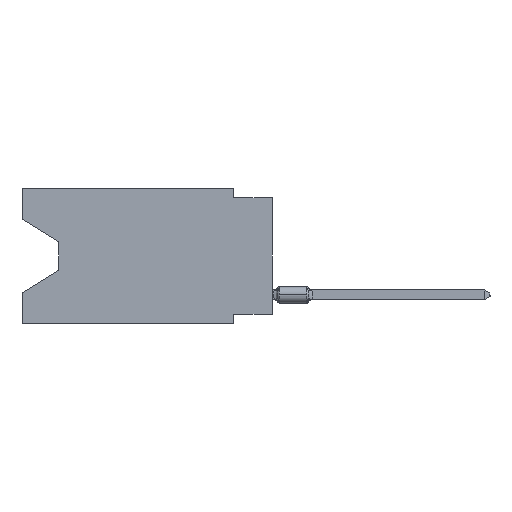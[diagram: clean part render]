
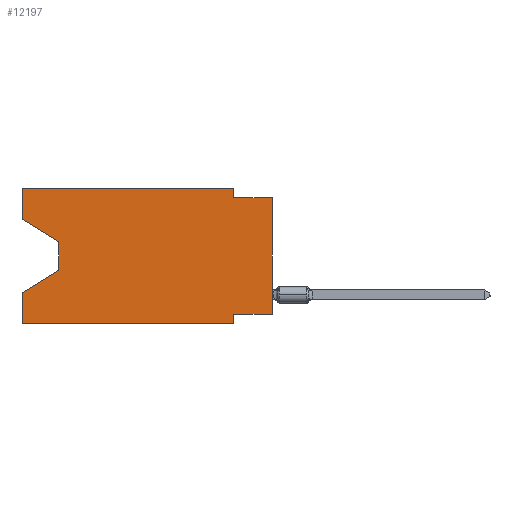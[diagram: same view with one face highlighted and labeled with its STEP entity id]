
A CAD part, left-side view. The second image highlights one B-rep face of the part: STEP entity #12197.
In plain terms, the highlighted planar face has unit normal (-1, 0, 0).
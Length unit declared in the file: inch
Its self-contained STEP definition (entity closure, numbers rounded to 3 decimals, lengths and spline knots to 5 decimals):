
#120 = CARTESIAN_POINT ( 'NONE',  ( 0., 0.645, 0. ) ) ;
#239 = VERTEX_POINT ( 'NONE', #30306 ) ;
#517 = FACE_OUTER_BOUND ( 'NONE', #9209, .T. ) ;
#869 = ORIENTED_EDGE ( 'NONE', *, *, #15282, .T. ) ;
#912 = DIRECTION ( 'NONE',  ( 0., 1., 0. ) ) ;
#1677 = DIRECTION ( 'NONE',  ( 0., 0., -1. ) ) ;
#1765 = VECTOR ( 'NONE', #13354, 39.37008 ) ;
#1964 = CARTESIAN_POINT ( 'NONE',  ( 0., 0.645, -0.08025 ) ) ;
#2589 = ORIENTED_EDGE ( 'NONE', *, *, #3923, .F. ) ;
#2932 = DIRECTION ( 'NONE',  ( 0., 0., 1. ) ) ;
#3113 = DIRECTION ( 'NONE',  ( 1., 0., 0. ) ) ;
#3173 = ORIENTED_EDGE ( 'NONE', *, *, #23445, .T. ) ;
#3202 = CARTESIAN_POINT ( 'NONE',  ( 0., 0.645, 0. ) ) ;
#3367 = LINE ( 'NONE', #14789, #26291 ) ;
#3440 = EDGE_CURVE ( 'NONE', #21007, #14443, #19970, .T. ) ;
#3761 = VECTOR ( 'NONE', #20895, 39.37008 ) ;
#3923 = EDGE_CURVE ( 'NONE', #27472, #8868, #16144, .T. ) ;
#5024 = ORIENTED_EDGE ( 'NONE', *, *, #17953, .T. ) ;
#5385 = CARTESIAN_POINT ( 'NONE',  ( 0., 0.1, -0.35 ) ) ;
#6150 = LINE ( 'NONE', #11535, #6259 ) ;
#6226 = CARTESIAN_POINT ( 'NONE',  ( 0., 0.55, -0.212 ) ) ;
#6236 = VECTOR ( 'NONE', #27005, 39.37008 ) ;
#6259 = VECTOR ( 'NONE', #1677, 39.37008 ) ;
#6413 = DIRECTION ( 'NONE',  ( 0., -1., 0. ) ) ;
#7606 = LINE ( 'NONE', #14845, #24814 ) ;
#8752 = VERTEX_POINT ( 'NONE', #9544 ) ;
#8868 = VERTEX_POINT ( 'NONE', #14634 ) ;
#9046 = DIRECTION ( 'NONE',  ( 0., -0.855, -0.519 ) ) ;
#9209 = EDGE_LOOP ( 'NONE', ( #3173, #12405, #17826, #14183, #869, #27420, #13983, #5024, #28191, #11538, #2589, #18697 ) ) ;
#9544 = CARTESIAN_POINT ( 'NONE',  ( 0., 0.1, -0.325 ) ) ;
#9711 = EDGE_CURVE ( 'NONE', #22845, #14443, #29004, .T. ) ;
#9905 = DIRECTION ( 'NONE',  ( 0., 0., -1. ) ) ;
#10498 = CARTESIAN_POINT ( 'NONE',  ( 0., 0., -0.325 ) ) ;
#10618 = CARTESIAN_POINT ( 'NONE',  ( 0., 0.645, 0. ) ) ;
#11204 = AXIS2_PLACEMENT_3D ( 'NONE', #24268, #3113, #9905 ) ;
#11452 = LINE ( 'NONE', #13619, #3761 ) ;
#11535 = CARTESIAN_POINT ( 'NONE',  ( 0., 0.55, -0.138 ) ) ;
#11538 = ORIENTED_EDGE ( 'NONE', *, *, #17455, .F. ) ;
#12197 = ADVANCED_FACE ( 'NONE', ( #517 ), #17171, .F. ) ;
#12328 = LINE ( 'NONE', #17131, #15081 ) ;
#12405 = ORIENTED_EDGE ( 'NONE', *, *, #18213, .T. ) ;
#13354 = DIRECTION ( 'NONE',  ( 0., 0., -1. ) ) ;
#13619 = CARTESIAN_POINT ( 'NONE',  ( 0., 0., -0.025 ) ) ;
#13983 = ORIENTED_EDGE ( 'NONE', *, *, #27570, .F. ) ;
#14183 = ORIENTED_EDGE ( 'NONE', *, *, #9711, .F. ) ;
#14443 = VERTEX_POINT ( 'NONE', #19877 ) ;
#14579 = VERTEX_POINT ( 'NONE', #26303 ) ;
#14634 = CARTESIAN_POINT ( 'NONE',  ( 0., 0.1, 0. ) ) ;
#14789 = CARTESIAN_POINT ( 'NONE',  ( 0., 0., -0.325 ) ) ;
#14845 = CARTESIAN_POINT ( 'NONE',  ( 0., 0.645, -0.35 ) ) ;
#15081 = VECTOR ( 'NONE', #2932, 39.37008 ) ;
#15213 = EDGE_CURVE ( 'NONE', #8752, #26318, #23974, .T. ) ;
#15282 = EDGE_CURVE ( 'NONE', #22845, #26318, #7606, .T. ) ;
#15330 = DIRECTION ( 'NONE',  ( 0., 0.855, -0.519 ) ) ;
#15989 = LINE ( 'NONE', #25106, #1765 ) ;
#16144 = LINE ( 'NONE', #25564, #18585 ) ;
#16969 = VECTOR ( 'NONE', #30060, 39.37008 ) ;
#17131 = CARTESIAN_POINT ( 'NONE',  ( 0., 0., 0. ) ) ;
#17171 = PLANE ( 'NONE',  #11204 ) ;
#17455 = EDGE_CURVE ( 'NONE', #8868, #25025, #15989, .T. ) ;
#17802 = CARTESIAN_POINT ( 'NONE',  ( 0., 0., -0.025 ) ) ;
#17826 = ORIENTED_EDGE ( 'NONE', *, *, #3440, .T. ) ;
#17953 = EDGE_CURVE ( 'NONE', #20462, #28483, #12328, .T. ) ;
#18213 = EDGE_CURVE ( 'NONE', #14579, #21007, #6150, .T. ) ;
#18585 = VECTOR ( 'NONE', #6413, 39.37008 ) ;
#18697 = ORIENTED_EDGE ( 'NONE', *, *, #26613, .F. ) ;
#19877 = CARTESIAN_POINT ( 'NONE',  ( 0., 0.645, -0.26975 ) ) ;
#19970 = LINE ( 'NONE', #6226, #24946 ) ;
#20462 = VERTEX_POINT ( 'NONE', #10498 ) ;
#20895 = DIRECTION ( 'NONE',  ( 0., -1., 0. ) ) ;
#21007 = VERTEX_POINT ( 'NONE', #22892 ) ;
#21113 = EDGE_CURVE ( 'NONE', #25025, #28483, #11452, .T. ) ;
#22524 = VECTOR ( 'NONE', #9046, 39.37008 ) ;
#22845 = VERTEX_POINT ( 'NONE', #23919 ) ;
#22892 = CARTESIAN_POINT ( 'NONE',  ( 0., 0.55, -0.212 ) ) ;
#23445 = EDGE_CURVE ( 'NONE', #239, #14579, #24945, .T. ) ;
#23919 = CARTESIAN_POINT ( 'NONE',  ( 0., 0.645, -0.35 ) ) ;
#23974 = LINE ( 'NONE', #24422, #26272 ) ;
#24268 = CARTESIAN_POINT ( 'NONE',  ( 0., 0.645, 0. ) ) ;
#24422 = CARTESIAN_POINT ( 'NONE',  ( 0., 0.1, -0.35 ) ) ;
#24814 = VECTOR ( 'NONE', #26592, 39.37008 ) ;
#24945 = LINE ( 'NONE', #1964, #22524 ) ;
#24946 = VECTOR ( 'NONE', #15330, 39.37008 ) ;
#25025 = VERTEX_POINT ( 'NONE', #26488 ) ;
#25106 = CARTESIAN_POINT ( 'NONE',  ( 0., 0.1, 0. ) ) ;
#25429 = LINE ( 'NONE', #120, #16969 ) ;
#25564 = CARTESIAN_POINT ( 'NONE',  ( 0., 0.645, 0. ) ) ;
#26272 = VECTOR ( 'NONE', #28890, 39.37008 ) ;
#26291 = VECTOR ( 'NONE', #912, 39.37008 ) ;
#26303 = CARTESIAN_POINT ( 'NONE',  ( 0., 0.55, -0.138 ) ) ;
#26318 = VERTEX_POINT ( 'NONE', #5385 ) ;
#26488 = CARTESIAN_POINT ( 'NONE',  ( 0., 0.1, -0.025 ) ) ;
#26592 = DIRECTION ( 'NONE',  ( 0., -1., 0. ) ) ;
#26613 = EDGE_CURVE ( 'NONE', #239, #27472, #25429, .T. ) ;
#27005 = DIRECTION ( 'NONE',  ( 0., 0., 1. ) ) ;
#27420 = ORIENTED_EDGE ( 'NONE', *, *, #15213, .F. ) ;
#27472 = VERTEX_POINT ( 'NONE', #3202 ) ;
#27570 = EDGE_CURVE ( 'NONE', #20462, #8752, #3367, .T. ) ;
#28191 = ORIENTED_EDGE ( 'NONE', *, *, #21113, .F. ) ;
#28483 = VERTEX_POINT ( 'NONE', #17802 ) ;
#28890 = DIRECTION ( 'NONE',  ( 0., 0., -1. ) ) ;
#29004 = LINE ( 'NONE', #10618, #6236 ) ;
#30060 = DIRECTION ( 'NONE',  ( 0., 0., 1. ) ) ;
#30306 = CARTESIAN_POINT ( 'NONE',  ( 0., 0.645, -0.08025 ) ) ;
